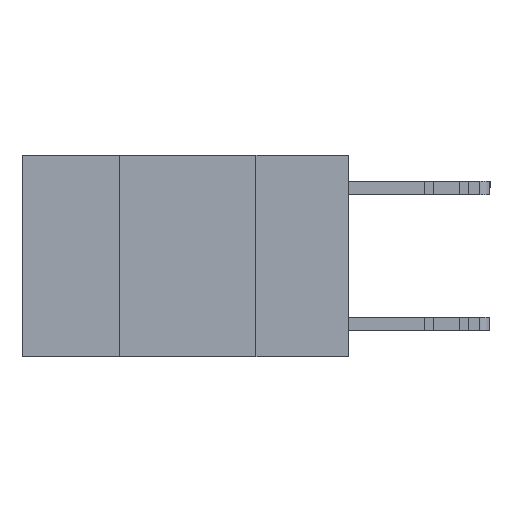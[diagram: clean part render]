
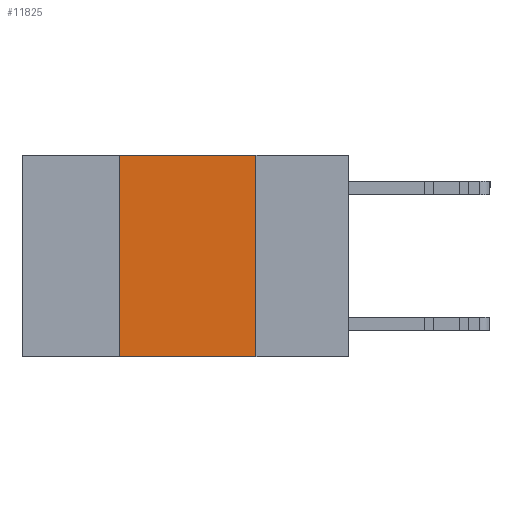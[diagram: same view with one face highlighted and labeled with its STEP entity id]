
A CAD part, left-side view. The second image highlights one B-rep face of the part: STEP entity #11825.
In plain terms, the highlighted planar face has unit normal (-1, 0, 0).
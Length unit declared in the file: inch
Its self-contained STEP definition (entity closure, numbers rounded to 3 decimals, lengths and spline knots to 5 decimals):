
#448 = ORIENTED_EDGE ( 'NONE', *, *, #20567, .F. ) ;
#1129 = DIRECTION ( 'NONE',  ( 0., -1., 0. ) ) ;
#1629 = EDGE_CURVE ( 'NONE', #12737, #26445, #2135, .T. ) ;
#2135 = LINE ( 'NONE', #7162, #15161 ) ;
#2981 = CARTESIAN_POINT ( 'NONE',  ( 0., 0.6, -0.37 ) ) ;
#3736 = EDGE_CURVE ( 'NONE', #28669, #29729, #7608, .T. ) ;
#7162 = CARTESIAN_POINT ( 'NONE',  ( 0., 0.17, 0. ) ) ;
#7608 = LINE ( 'NONE', #12618, #25672 ) ;
#8294 = LINE ( 'NONE', #17591, #29378 ) ;
#9746 = DIRECTION ( 'NONE',  ( 0., 0., -1. ) ) ;
#9838 = LINE ( 'NONE', #2981, #11054 ) ;
#11035 = CARTESIAN_POINT ( 'NONE',  ( 0., 0.17, 0. ) ) ;
#11054 = VECTOR ( 'NONE', #26762, 39.37008 ) ;
#11394 = CARTESIAN_POINT ( 'NONE',  ( 0., 0.6, 0. ) ) ;
#11825 = ADVANCED_FACE ( 'NONE', ( #17856 ), #19695, .F. ) ;
#12567 = CARTESIAN_POINT ( 'NONE',  ( 0., 0.17, -0.37 ) ) ;
#12618 = CARTESIAN_POINT ( 'NONE',  ( 0., 0.42, 0. ) ) ;
#12737 = VERTEX_POINT ( 'NONE', #11035 ) ;
#13331 = ORIENTED_EDGE ( 'NONE', *, *, #1629, .F. ) ;
#14987 = CARTESIAN_POINT ( 'NONE',  ( 0., 0.42, -0.37 ) ) ;
#15161 = VECTOR ( 'NONE', #9746, 39.37008 ) ;
#16515 = ORIENTED_EDGE ( 'NONE', *, *, #26490, .T. ) ;
#16890 = DIRECTION ( 'NONE',  ( 0., 0., 1. ) ) ;
#17591 = CARTESIAN_POINT ( 'NONE',  ( 0., 0.6, 0. ) ) ;
#17856 = FACE_OUTER_BOUND ( 'NONE', #25700, .T. ) ;
#19271 = AXIS2_PLACEMENT_3D ( 'NONE', #11394, #27008, #27155 ) ;
#19695 = PLANE ( 'NONE',  #19271 ) ;
#20567 = EDGE_CURVE ( 'NONE', #29729, #12737, #8294, .T. ) ;
#25672 = VECTOR ( 'NONE', #16890, 39.37008 ) ;
#25700 = EDGE_LOOP ( 'NONE', ( #13331, #448, #28596, #16515 ) ) ;
#26445 = VERTEX_POINT ( 'NONE', #12567 ) ;
#26490 = EDGE_CURVE ( 'NONE', #28669, #26445, #9838, .T. ) ;
#26762 = DIRECTION ( 'NONE',  ( 0., -1., 0. ) ) ;
#27008 = DIRECTION ( 'NONE',  ( 1., 0., 0. ) ) ;
#27155 = DIRECTION ( 'NONE',  ( 0., 0., -1. ) ) ;
#28596 = ORIENTED_EDGE ( 'NONE', *, *, #3736, .F. ) ;
#28669 = VERTEX_POINT ( 'NONE', #14987 ) ;
#29378 = VECTOR ( 'NONE', #1129, 39.37008 ) ;
#29729 = VERTEX_POINT ( 'NONE', #30080 ) ;
#30080 = CARTESIAN_POINT ( 'NONE',  ( 0., 0.42, 0. ) ) ;
